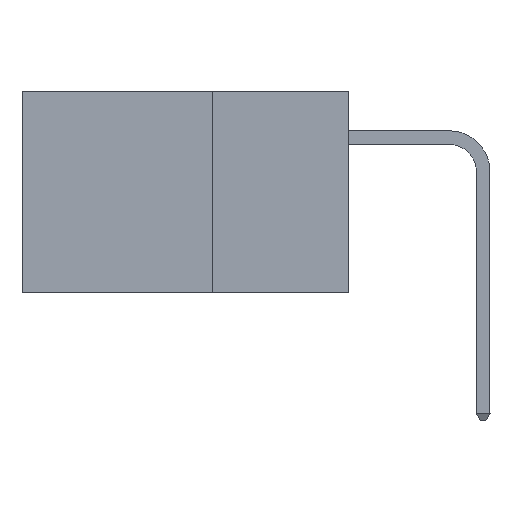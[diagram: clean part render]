
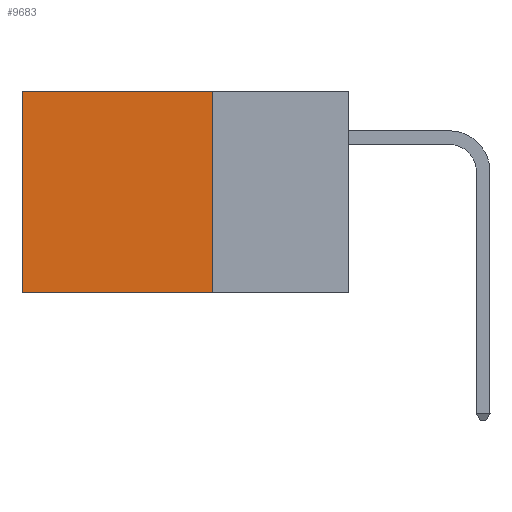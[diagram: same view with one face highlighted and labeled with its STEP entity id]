
A CAD part, left-side view. The second image highlights one B-rep face of the part: STEP entity #9683.
In plain terms, the highlighted planar face has unit normal (-1, 0, 0).
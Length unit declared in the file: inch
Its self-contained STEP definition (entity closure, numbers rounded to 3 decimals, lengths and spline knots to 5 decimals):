
#361 = CARTESIAN_POINT ( 'NONE',  ( 0.2875, 0.6, 0. ) ) ;
#1453 = VERTEX_POINT ( 'NONE', #15102 ) ;
#3578 = LINE ( 'NONE', #15405, #14377 ) ;
#4000 = CARTESIAN_POINT ( 'NONE',  ( 0.2875, 0.25, 0. ) ) ;
#4022 = EDGE_LOOP ( 'NONE', ( #17326, #11175, #15466, #10611 ) ) ;
#5036 = PLANE ( 'NONE',  #16848 ) ;
#6419 = DIRECTION ( 'NONE',  ( 0., 1., 0. ) ) ;
#6615 = EDGE_CURVE ( 'NONE', #12390, #14524, #14639, .T. ) ;
#8102 = DIRECTION ( 'NONE',  ( 0., 0., -1. ) ) ;
#8744 = FACE_OUTER_BOUND ( 'NONE', #4022, .T. ) ;
#9683 = ADVANCED_FACE ( 'NONE', ( #8744 ), #5036, .F. ) ;
#10611 = ORIENTED_EDGE ( 'NONE', *, *, #20226, .T. ) ;
#11175 = ORIENTED_EDGE ( 'NONE', *, *, #11758, .F. ) ;
#11377 = VECTOR ( 'NONE', #17573, 39.37008 ) ;
#11758 = EDGE_CURVE ( 'NONE', #14524, #1453, #3578, .T. ) ;
#12390 = VERTEX_POINT ( 'NONE', #4000 ) ;
#13397 = LINE ( 'NONE', #14863, #14594 ) ;
#13537 = CARTESIAN_POINT ( 'NONE',  ( 0.2875, 0.6, 0. ) ) ;
#13593 = DIRECTION ( 'NONE',  ( 1., 0., 0. ) ) ;
#14377 = VECTOR ( 'NONE', #16967, 39.37008 ) ;
#14524 = VERTEX_POINT ( 'NONE', #17333 ) ;
#14594 = VECTOR ( 'NONE', #6419, 39.37008 ) ;
#14639 = LINE ( 'NONE', #21489, #16102 ) ;
#14863 = CARTESIAN_POINT ( 'NONE',  ( 0.2875, 0.25, 0. ) ) ;
#15102 = CARTESIAN_POINT ( 'NONE',  ( 0.2875, 0.6, -0.37 ) ) ;
#15165 = CARTESIAN_POINT ( 'NONE',  ( 0.2875, 0.25, 0. ) ) ;
#15405 = CARTESIAN_POINT ( 'NONE',  ( 0.2875, 0.25, -0.37 ) ) ;
#15466 = ORIENTED_EDGE ( 'NONE', *, *, #6615, .F. ) ;
#15892 = LINE ( 'NONE', #361, #11377 ) ;
#16102 = VECTOR ( 'NONE', #8102, 39.37008 ) ;
#16645 = VERTEX_POINT ( 'NONE', #13537 ) ;
#16848 = AXIS2_PLACEMENT_3D ( 'NONE', #15165, #13593, #20325 ) ;
#16967 = DIRECTION ( 'NONE',  ( 0., 1., 0. ) ) ;
#17326 = ORIENTED_EDGE ( 'NONE', *, *, #21140, .T. ) ;
#17333 = CARTESIAN_POINT ( 'NONE',  ( 0.2875, 0.25, -0.37 ) ) ;
#17573 = DIRECTION ( 'NONE',  ( 0., 0., -1. ) ) ;
#20226 = EDGE_CURVE ( 'NONE', #12390, #16645, #13397, .T. ) ;
#20325 = DIRECTION ( 'NONE',  ( 0., 0., -1. ) ) ;
#21140 = EDGE_CURVE ( 'NONE', #16645, #1453, #15892, .T. ) ;
#21489 = CARTESIAN_POINT ( 'NONE',  ( 0.2875, 0.25, 0. ) ) ;
